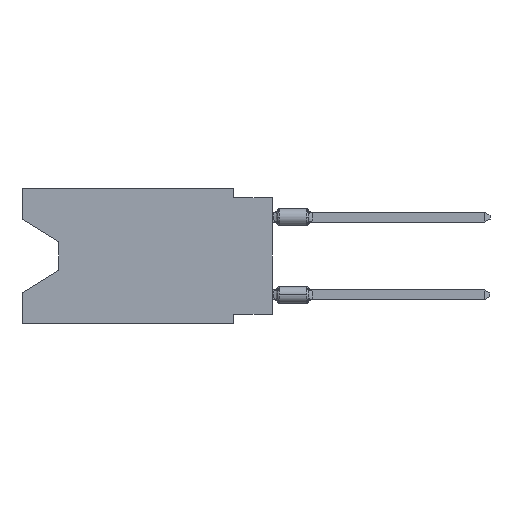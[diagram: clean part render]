
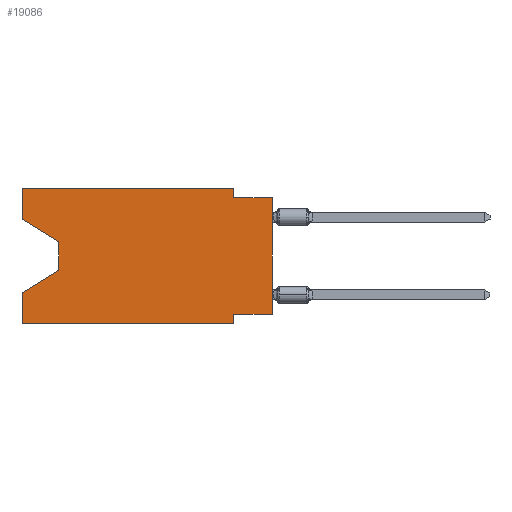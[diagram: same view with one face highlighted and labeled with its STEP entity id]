
A CAD part, left-side view. The second image highlights one B-rep face of the part: STEP entity #19086.
In plain terms, the highlighted planar face has unit normal (-1, 0, 0).
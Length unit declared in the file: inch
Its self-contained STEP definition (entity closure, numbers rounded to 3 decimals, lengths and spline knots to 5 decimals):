
#37 = ORIENTED_EDGE ( 'NONE', *, *, #23125, .F. ) ;
#48 = DIRECTION ( 'NONE',  ( 0., -1., 0. ) ) ;
#904 = EDGE_LOOP ( 'NONE', ( #21496, #13659, #6398, #24169, #19833, #6264, #16674, #18608, #20957, #2172, #8195, #37 ) ) ;
#913 = VECTOR ( 'NONE', #1203, 39.37008 ) ;
#931 = DIRECTION ( 'NONE',  ( 0., 0.855, -0.519 ) ) ;
#1203 = DIRECTION ( 'NONE',  ( 0., 1., 0. ) ) ;
#1421 = VECTOR ( 'NONE', #15816, 39.37008 ) ;
#1572 = EDGE_CURVE ( 'NONE', #12703, #10358, #15946, .T. ) ;
#1794 = VECTOR ( 'NONE', #48, 39.37008 ) ;
#1908 = EDGE_CURVE ( 'NONE', #12367, #12703, #23132, .T. ) ;
#2172 = ORIENTED_EDGE ( 'NONE', *, *, #20023, .F. ) ;
#2177 = VERTEX_POINT ( 'NONE', #14038 ) ;
#2349 = CARTESIAN_POINT ( 'NONE',  ( 0., 0.645, 0. ) ) ;
#2429 = DIRECTION ( 'NONE',  ( 0., 0., -1. ) ) ;
#2451 = DIRECTION ( 'NONE',  ( 0., -1., 0. ) ) ;
#2541 = CARTESIAN_POINT ( 'NONE',  ( 0., 0.645, 0. ) ) ;
#2559 = CARTESIAN_POINT ( 'NONE',  ( 0., 0., -0.025 ) ) ;
#2583 = VECTOR ( 'NONE', #3991, 39.37008 ) ;
#2608 = CARTESIAN_POINT ( 'NONE',  ( 0., 0.645, 0. ) ) ;
#2973 = VECTOR ( 'NONE', #6617, 39.37008 ) ;
#3991 = DIRECTION ( 'NONE',  ( 0., 0., -1. ) ) ;
#4126 = DIRECTION ( 'NONE',  ( 0., 0., -1. ) ) ;
#4191 = LINE ( 'NONE', #2559, #1421 ) ;
#4218 = EDGE_CURVE ( 'NONE', #8566, #21850, #18934, .T. ) ;
#4469 = FACE_OUTER_BOUND ( 'NONE', #904, .T. ) ;
#5115 = VERTEX_POINT ( 'NONE', #11253 ) ;
#5150 = CARTESIAN_POINT ( 'NONE',  ( 0., 0.55, -0.212 ) ) ;
#5219 = DIRECTION ( 'NONE',  ( 0., 0., -1. ) ) ;
#5259 = CARTESIAN_POINT ( 'NONE',  ( 0., 0., -0.025 ) ) ;
#5595 = CARTESIAN_POINT ( 'NONE',  ( 0., 0.1, 0. ) ) ;
#6264 = ORIENTED_EDGE ( 'NONE', *, *, #7590, .F. ) ;
#6398 = ORIENTED_EDGE ( 'NONE', *, *, #1572, .T. ) ;
#6617 = DIRECTION ( 'NONE',  ( 0., 0., 1. ) ) ;
#6892 = CARTESIAN_POINT ( 'NONE',  ( 0., 0.645, -0.35 ) ) ;
#6905 = VECTOR ( 'NONE', #931, 39.37008 ) ;
#7590 = EDGE_CURVE ( 'NONE', #5115, #21850, #11606, .T. ) ;
#7828 = CARTESIAN_POINT ( 'NONE',  ( 0., 0., 0. ) ) ;
#8195 = ORIENTED_EDGE ( 'NONE', *, *, #23997, .F. ) ;
#8566 = VERTEX_POINT ( 'NONE', #6892 ) ;
#9013 = VECTOR ( 'NONE', #22149, 39.37008 ) ;
#9138 = VERTEX_POINT ( 'NONE', #17325 ) ;
#10358 = VERTEX_POINT ( 'NONE', #24663 ) ;
#10435 = CARTESIAN_POINT ( 'NONE',  ( 0., 0.55, -0.212 ) ) ;
#10453 = CARTESIAN_POINT ( 'NONE',  ( 0., 0.645, -0.08025 ) ) ;
#11216 = CARTESIAN_POINT ( 'NONE',  ( 0., 0.1, -0.35 ) ) ;
#11253 = CARTESIAN_POINT ( 'NONE',  ( 0., 0.1, -0.325 ) ) ;
#11606 = LINE ( 'NONE', #13133, #2583 ) ;
#12094 = PLANE ( 'NONE',  #20943 ) ;
#12367 = VERTEX_POINT ( 'NONE', #19157 ) ;
#12703 = VERTEX_POINT ( 'NONE', #5150 ) ;
#12811 = VERTEX_POINT ( 'NONE', #5259 ) ;
#12886 = CARTESIAN_POINT ( 'NONE',  ( 0., 0.645, 0. ) ) ;
#13100 = DIRECTION ( 'NONE',  ( 1., 0., 0. ) ) ;
#13133 = CARTESIAN_POINT ( 'NONE',  ( 0., 0.1, -0.35 ) ) ;
#13425 = VECTOR ( 'NONE', #24694, 39.37008 ) ;
#13659 = ORIENTED_EDGE ( 'NONE', *, *, #1908, .T. ) ;
#14038 = CARTESIAN_POINT ( 'NONE',  ( 0., 0.1, -0.025 ) ) ;
#14114 = CARTESIAN_POINT ( 'NONE',  ( 0., 0.55, -0.138 ) ) ;
#14816 = CARTESIAN_POINT ( 'NONE',  ( 0., 0.645, -0.35 ) ) ;
#15202 = LINE ( 'NONE', #19574, #20206 ) ;
#15816 = DIRECTION ( 'NONE',  ( 0., -1., 0. ) ) ;
#15946 = LINE ( 'NONE', #10435, #6905 ) ;
#16674 = ORIENTED_EDGE ( 'NONE', *, *, #17502, .F. ) ;
#16703 = VERTEX_POINT ( 'NONE', #10453 ) ;
#16977 = EDGE_CURVE ( 'NONE', #16703, #12367, #23428, .T. ) ;
#17325 = CARTESIAN_POINT ( 'NONE',  ( 0., 0., -0.325 ) ) ;
#17502 = EDGE_CURVE ( 'NONE', #9138, #5115, #18583, .T. ) ;
#17585 = LINE ( 'NONE', #2349, #2973 ) ;
#18583 = LINE ( 'NONE', #23692, #913 ) ;
#18608 = ORIENTED_EDGE ( 'NONE', *, *, #24370, .T. ) ;
#18934 = LINE ( 'NONE', #14816, #1794 ) ;
#19018 = VECTOR ( 'NONE', #4126, 39.37008 ) ;
#19086 = ADVANCED_FACE ( 'NONE', ( #4469 ), #12094, .F. ) ;
#19157 = CARTESIAN_POINT ( 'NONE',  ( 0., 0.55, -0.138 ) ) ;
#19184 = CARTESIAN_POINT ( 'NONE',  ( 0., 0.1, 0. ) ) ;
#19574 = CARTESIAN_POINT ( 'NONE',  ( 0., 0.645, 0. ) ) ;
#19667 = CARTESIAN_POINT ( 'NONE',  ( 0., 0.645, -0.08025 ) ) ;
#19672 = LINE ( 'NONE', #19184, #20984 ) ;
#19833 = ORIENTED_EDGE ( 'NONE', *, *, #4218, .T. ) ;
#19947 = EDGE_CURVE ( 'NONE', #2177, #12811, #4191, .T. ) ;
#20023 = EDGE_CURVE ( 'NONE', #21830, #2177, #19672, .T. ) ;
#20206 = VECTOR ( 'NONE', #2451, 39.37008 ) ;
#20647 = LINE ( 'NONE', #12886, #9013 ) ;
#20722 = EDGE_CURVE ( 'NONE', #8566, #10358, #17585, .T. ) ;
#20943 = AXIS2_PLACEMENT_3D ( 'NONE', #2608, #13100, #5219 ) ;
#20957 = ORIENTED_EDGE ( 'NONE', *, *, #19947, .F. ) ;
#20984 = VECTOR ( 'NONE', #2429, 39.37008 ) ;
#21188 = LINE ( 'NONE', #7828, #13425 ) ;
#21496 = ORIENTED_EDGE ( 'NONE', *, *, #16977, .T. ) ;
#21680 = DIRECTION ( 'NONE',  ( 0., -0.855, -0.519 ) ) ;
#21830 = VERTEX_POINT ( 'NONE', #5595 ) ;
#21850 = VERTEX_POINT ( 'NONE', #11216 ) ;
#22149 = DIRECTION ( 'NONE',  ( 0., 0., 1. ) ) ;
#22583 = VERTEX_POINT ( 'NONE', #2541 ) ;
#23125 = EDGE_CURVE ( 'NONE', #16703, #22583, #20647, .T. ) ;
#23132 = LINE ( 'NONE', #14114, #19018 ) ;
#23428 = LINE ( 'NONE', #19667, #23636 ) ;
#23636 = VECTOR ( 'NONE', #21680, 39.37008 ) ;
#23692 = CARTESIAN_POINT ( 'NONE',  ( 0., 0., -0.325 ) ) ;
#23997 = EDGE_CURVE ( 'NONE', #22583, #21830, #15202, .T. ) ;
#24169 = ORIENTED_EDGE ( 'NONE', *, *, #20722, .F. ) ;
#24370 = EDGE_CURVE ( 'NONE', #9138, #12811, #21188, .T. ) ;
#24663 = CARTESIAN_POINT ( 'NONE',  ( 0., 0.645, -0.26975 ) ) ;
#24694 = DIRECTION ( 'NONE',  ( 0., 0., 1. ) ) ;
